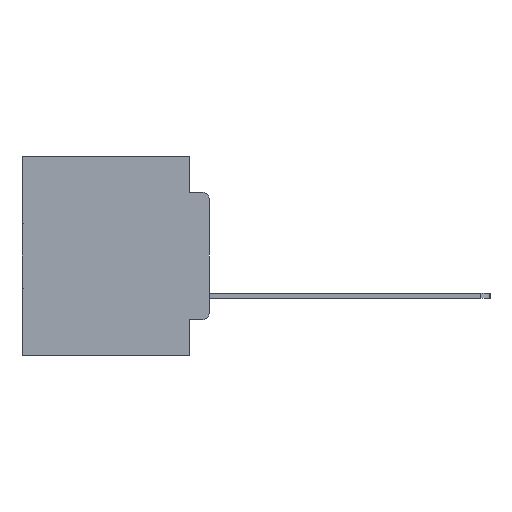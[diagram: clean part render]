
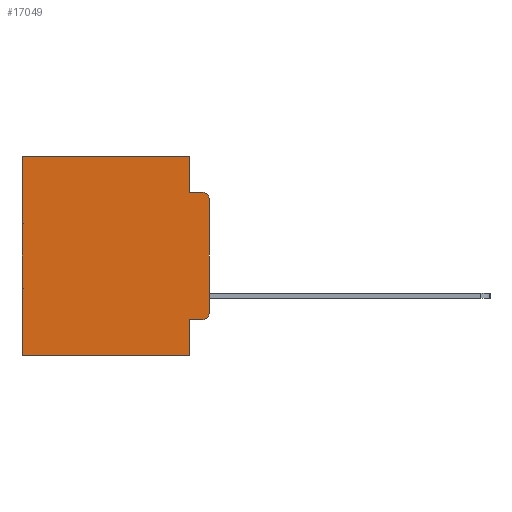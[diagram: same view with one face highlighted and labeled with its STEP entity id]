
A CAD part, left-side view. The second image highlights one B-rep face of the part: STEP entity #17049.
In plain terms, the highlighted planar face has unit normal (-1, 0, 0).
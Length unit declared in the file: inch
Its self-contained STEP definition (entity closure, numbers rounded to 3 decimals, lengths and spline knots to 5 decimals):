
#474 = EDGE_CURVE ( 'NONE', #28206, #2827, #13190, .T. ) ;
#853 = FACE_OUTER_BOUND ( 'NONE', #31362, .T. ) ;
#1542 = EDGE_CURVE ( 'NONE', #19422, #19389, #3302, .T. ) ;
#1835 = LINE ( 'NONE', #17226, #14396 ) ;
#1882 = LINE ( 'NONE', #5799, #20970 ) ;
#2091 = DIRECTION ( 'NONE',  ( 0., 0., -1. ) ) ;
#2380 = CARTESIAN_POINT ( 'NONE',  ( 0.298, 0.051, -0.0885 ) ) ;
#2827 = VERTEX_POINT ( 'NONE', #10625 ) ;
#3067 = DIRECTION ( 'NONE',  ( 0., 1., 0. ) ) ;
#3071 = ORIENTED_EDGE ( 'NONE', *, *, #30704, .T. ) ;
#3267 = VERTEX_POINT ( 'NONE', #11684 ) ;
#3302 = LINE ( 'NONE', #6287, #21575 ) ;
#3750 = VERTEX_POINT ( 'NONE', #23466 ) ;
#3796 = VERTEX_POINT ( 'NONE', #18302 ) ;
#5799 = CARTESIAN_POINT ( 'NONE',  ( 0.298, 0.051, 0. ) ) ;
#6287 = CARTESIAN_POINT ( 'NONE',  ( 0.298, 0., 0. ) ) ;
#6813 = ORIENTED_EDGE ( 'NONE', *, *, #14812, .F. ) ;
#7180 = CARTESIAN_POINT ( 'NONE',  ( 0.298, 0.02, -0.0885 ) ) ;
#7235 = EDGE_CURVE ( 'NONE', #26424, #3750, #30743, .T. ) ;
#7337 = ORIENTED_EDGE ( 'NONE', *, *, #1542, .F. ) ;
#8068 = VECTOR ( 'NONE', #20927, 39.37008 ) ;
#8318 = EDGE_CURVE ( 'NONE', #3267, #26424, #31774, .T. ) ;
#8492 = DIRECTION ( 'NONE',  ( 0., 1., 0. ) ) ;
#8897 = EDGE_CURVE ( 'NONE', #3267, #12263, #1882, .T. ) ;
#9189 = DIRECTION ( 'NONE',  ( -1., 0., 0. ) ) ;
#9415 = AXIS2_PLACEMENT_3D ( 'NONE', #31405, #17065, #2091 ) ;
#9718 = CARTESIAN_POINT ( 'NONE',  ( 0.298, 0., -0.3915 ) ) ;
#10625 = CARTESIAN_POINT ( 'NONE',  ( 0.298, 0.051, -0.5 ) ) ;
#11684 = CARTESIAN_POINT ( 'NONE',  ( 0.298, 0.051, 0. ) ) ;
#12019 = CARTESIAN_POINT ( 'NONE',  ( 0.298, 0.051, 0. ) ) ;
#12263 = VERTEX_POINT ( 'NONE', #2380 ) ;
#13190 = LINE ( 'NONE', #12019, #8068 ) ;
#13561 = CARTESIAN_POINT ( 'NONE',  ( 0.298, 0., 0. ) ) ;
#13668 = CARTESIAN_POINT ( 'NONE',  ( 0.298, 0.051, -0.4115 ) ) ;
#13960 = EDGE_CURVE ( 'NONE', #12263, #30936, #1835, .T. ) ;
#14396 = VECTOR ( 'NONE', #31553, 39.37008 ) ;
#14812 = EDGE_CURVE ( 'NONE', #2827, #3750, #30498, .T. ) ;
#14894 = DIRECTION ( 'NONE',  ( -1., 0., 0. ) ) ;
#15313 = ORIENTED_EDGE ( 'NONE', *, *, #8897, .F. ) ;
#15861 = ORIENTED_EDGE ( 'NONE', *, *, #7235, .T. ) ;
#15902 = ORIENTED_EDGE ( 'NONE', *, *, #13960, .F. ) ;
#15957 = AXIS2_PLACEMENT_3D ( 'NONE', #23951, #9189, #26360 ) ;
#16995 = VECTOR ( 'NONE', #3067, 39.37008 ) ;
#17049 = ADVANCED_FACE ( 'NONE', ( #853 ), #31303, .F. ) ;
#17065 = DIRECTION ( 'NONE',  ( 1., 0., 0. ) ) ;
#17099 = CARTESIAN_POINT ( 'NONE',  ( 0.298, 0.473, 0. ) ) ;
#17111 = CIRCLE ( 'NONE', #23648, 0.02 ) ;
#17226 = CARTESIAN_POINT ( 'NONE',  ( 0.298, 0.051, -0.0885 ) ) ;
#18302 = CARTESIAN_POINT ( 'NONE',  ( 0.298, 0.02, -0.4115 ) ) ;
#18916 = CARTESIAN_POINT ( 'NONE',  ( 0.298, 0.473, 0. ) ) ;
#18979 = ORIENTED_EDGE ( 'NONE', *, *, #474, .F. ) ;
#19016 = DIRECTION ( 'NONE',  ( 0., 0., -1. ) ) ;
#19115 = VECTOR ( 'NONE', #8492, 39.37008 ) ;
#19389 = VERTEX_POINT ( 'NONE', #9718 ) ;
#19422 = VERTEX_POINT ( 'NONE', #22160 ) ;
#20483 = CARTESIAN_POINT ( 'NONE',  ( 0.298, 0., -0.5 ) ) ;
#20516 = CIRCLE ( 'NONE', #15957, 0.02 ) ;
#20536 = ORIENTED_EDGE ( 'NONE', *, *, #8318, .T. ) ;
#20546 = EDGE_CURVE ( 'NONE', #19422, #30936, #20516, .T. ) ;
#20724 = DIRECTION ( 'NONE',  ( 0., 0., -1. ) ) ;
#20927 = DIRECTION ( 'NONE',  ( 0., 0., -1. ) ) ;
#20970 = VECTOR ( 'NONE', #20724, 39.37008 ) ;
#21075 = LINE ( 'NONE', #13668, #26708 ) ;
#21575 = VECTOR ( 'NONE', #26580, 39.37008 ) ;
#22160 = CARTESIAN_POINT ( 'NONE',  ( 0.298, 0., -0.1085 ) ) ;
#22452 = CARTESIAN_POINT ( 'NONE',  ( 0.298, 0.051, -0.4115 ) ) ;
#23466 = CARTESIAN_POINT ( 'NONE',  ( 0.298, 0.473, -0.5 ) ) ;
#23648 = AXIS2_PLACEMENT_3D ( 'NONE', #29360, #14894, #31700 ) ;
#23951 = CARTESIAN_POINT ( 'NONE',  ( 0.298, 0.02, -0.1085 ) ) ;
#24480 = VECTOR ( 'NONE', #19016, 39.37008 ) ;
#26360 = DIRECTION ( 'NONE',  ( 0., 0., -1. ) ) ;
#26424 = VERTEX_POINT ( 'NONE', #17099 ) ;
#26580 = DIRECTION ( 'NONE',  ( 0., 0., -1. ) ) ;
#26598 = ORIENTED_EDGE ( 'NONE', *, *, #27569, .T. ) ;
#26708 = VECTOR ( 'NONE', #30641, 39.37008 ) ;
#27569 = EDGE_CURVE ( 'NONE', #3796, #19389, #17111, .T. ) ;
#28206 = VERTEX_POINT ( 'NONE', #22452 ) ;
#29360 = CARTESIAN_POINT ( 'NONE',  ( 0.298, 0.02, -0.3915 ) ) ;
#29629 = ORIENTED_EDGE ( 'NONE', *, *, #20546, .T. ) ;
#30498 = LINE ( 'NONE', #20483, #16995 ) ;
#30641 = DIRECTION ( 'NONE',  ( 0., -1., 0. ) ) ;
#30704 = EDGE_CURVE ( 'NONE', #28206, #3796, #21075, .T. ) ;
#30743 = LINE ( 'NONE', #18916, #24480 ) ;
#30936 = VERTEX_POINT ( 'NONE', #7180 ) ;
#31303 = PLANE ( 'NONE',  #9415 ) ;
#31362 = EDGE_LOOP ( 'NONE', ( #7337, #29629, #15902, #15313, #20536, #15861, #6813, #18979, #3071, #26598 ) ) ;
#31405 = CARTESIAN_POINT ( 'NONE',  ( 0.298, 0., 0. ) ) ;
#31553 = DIRECTION ( 'NONE',  ( 0., -1., 0. ) ) ;
#31700 = DIRECTION ( 'NONE',  ( 0., 0., -1. ) ) ;
#31774 = LINE ( 'NONE', #13561, #19115 ) ;
